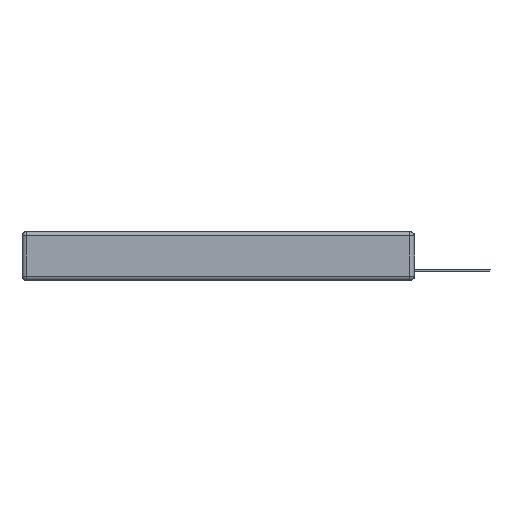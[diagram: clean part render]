
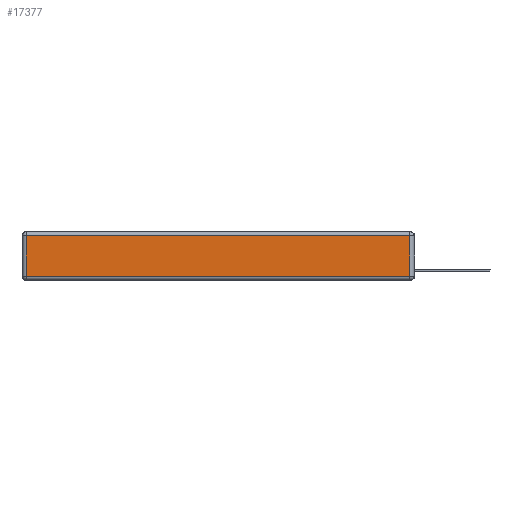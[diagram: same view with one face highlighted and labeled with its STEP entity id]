
A CAD part, left-side view. The second image highlights one B-rep face of the part: STEP entity #17377.
In plain terms, the highlighted planar face has unit normal (-1, 0, 0).
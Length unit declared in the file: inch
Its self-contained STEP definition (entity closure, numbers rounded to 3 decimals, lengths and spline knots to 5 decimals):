
#166 = ORIENTED_EDGE ( 'NONE', *, *, #6260, .T. ) ;
#1077 = VECTOR ( 'NONE', #5692, 39.37008 ) ;
#3736 = FACE_OUTER_BOUND ( 'NONE', #15926, .T. ) ;
#5414 = EDGE_CURVE ( 'NONE', #18390, #7665, #24001, .T. ) ;
#5692 = DIRECTION ( 'NONE',  ( 0., 1., 0. ) ) ;
#6260 = EDGE_CURVE ( 'NONE', #7665, #12961, #16500, .T. ) ;
#6751 = CARTESIAN_POINT ( 'NONE',  ( 0., 0.03, -0.03 ) ) ;
#6828 = CARTESIAN_POINT ( 'NONE',  ( 0., 2.72, -0.313 ) ) ;
#7623 = EDGE_CURVE ( 'NONE', #12961, #15013, #21038, .T. ) ;
#7665 = VERTEX_POINT ( 'NONE', #6828 ) ;
#8017 = ORIENTED_EDGE ( 'NONE', *, *, #5414, .T. ) ;
#9495 = DIRECTION ( 'NONE',  ( -1., 0., 0. ) ) ;
#9695 = VECTOR ( 'NONE', #24658, 39.37008 ) ;
#12553 = CARTESIAN_POINT ( 'NONE',  ( 0., 0.03, -0.313 ) ) ;
#12756 = PLANE ( 'NONE',  #19464 ) ;
#12961 = VERTEX_POINT ( 'NONE', #12553 ) ;
#14153 = VECTOR ( 'NONE', #22925, 39.37008 ) ;
#15013 = VERTEX_POINT ( 'NONE', #6751 ) ;
#15704 = CARTESIAN_POINT ( 'NONE',  ( 0., 2.75, -0.03 ) ) ;
#15926 = EDGE_LOOP ( 'NONE', ( #166, #16077, #19676, #8017 ) ) ;
#16077 = ORIENTED_EDGE ( 'NONE', *, *, #7623, .T. ) ;
#16500 = LINE ( 'NONE', #24539, #9695 ) ;
#17207 = CARTESIAN_POINT ( 'NONE',  ( 0., 2.72, -0.343 ) ) ;
#17377 = ADVANCED_FACE ( 'NONE', ( #3736 ), #12756, .T. ) ;
#18390 = VERTEX_POINT ( 'NONE', #21592 ) ;
#18791 = CARTESIAN_POINT ( 'NONE',  ( 0., 0., -0.343 ) ) ;
#19093 = DIRECTION ( 'NONE',  ( 0., 0., -1. ) ) ;
#19464 = AXIS2_PLACEMENT_3D ( 'NONE', #18791, #9495, #24692 ) ;
#19530 = EDGE_CURVE ( 'NONE', #15013, #18390, #22877, .T. ) ;
#19676 = ORIENTED_EDGE ( 'NONE', *, *, #19530, .T. ) ;
#21038 = LINE ( 'NONE', #24691, #14153 ) ;
#21592 = CARTESIAN_POINT ( 'NONE',  ( 0., 2.72, -0.03 ) ) ;
#22877 = LINE ( 'NONE', #15704, #1077 ) ;
#22900 = VECTOR ( 'NONE', #19093, 39.37008 ) ;
#22925 = DIRECTION ( 'NONE',  ( 0., 0., 1. ) ) ;
#24001 = LINE ( 'NONE', #17207, #22900 ) ;
#24539 = CARTESIAN_POINT ( 'NONE',  ( 0., 0., -0.313 ) ) ;
#24658 = DIRECTION ( 'NONE',  ( 0., -1., 0. ) ) ;
#24691 = CARTESIAN_POINT ( 'NONE',  ( 0., 0.03, -0.343 ) ) ;
#24692 = DIRECTION ( 'NONE',  ( 0., 0., 1. ) ) ;
